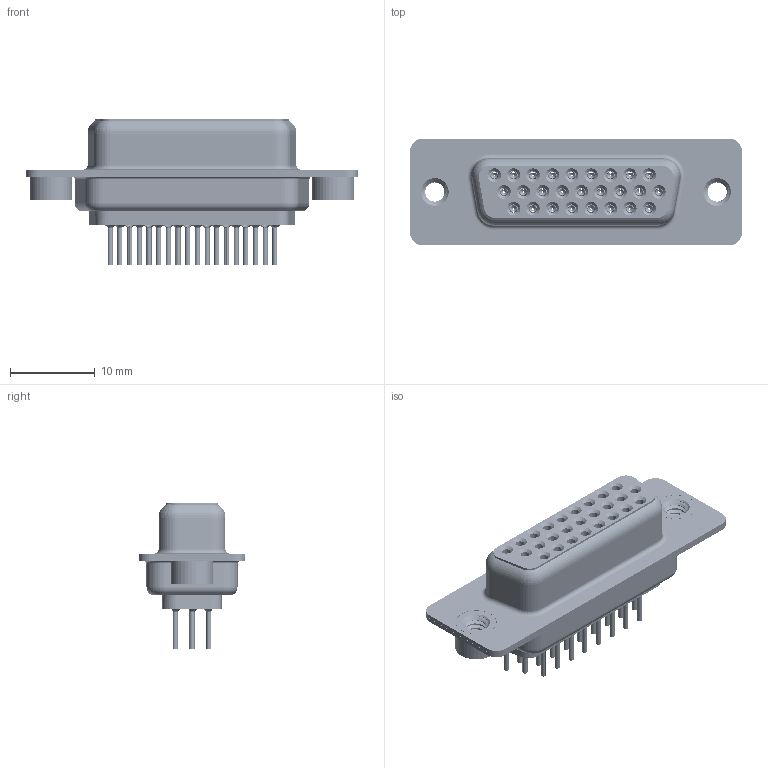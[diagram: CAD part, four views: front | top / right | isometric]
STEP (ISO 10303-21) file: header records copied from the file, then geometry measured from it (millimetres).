
FILE_DESCRIPTION (( 'STEP AP203' ), '1' );
FILE_NAME ('638-026-630-242.STEP', '2020-07-18T21:17:37', ( '' ), ( '' ), 'SwSTEP 2.0', 'SolidWorks 2020', '' );
FILE_SCHEMA (( 'CONFIG_CONTROL_DESIGN' ));
Length unit declared in the file: millimetre
Products named in the file (8): 638 Shell Rear_26 Contacts; 638 Housing_26 Contacts; 638 Contact Row 2_30; 638-026-630-242; 638 4-40 Threaded Rivet; 638 Contact Row 1_30; 638 Contact Row 3_30; 638 Shell Front_26 Contacts
Assembly tree (31 placements, depth 2):
  638-026-630-242
    638 Housing_26 Contacts
    638 Shell Front_26 Contacts
    638 Shell Rear_26 Contacts
    638 Contact Row 1_30  x9
    638 Contact Row 2_30  x9
    638 Contact Row 3_30  x8
    638 4-40 Threaded Rivet  x2
Bounding box: 39.19 x 12.6 x 17.3 mm (x, y, z)
Volume: 2214 mm3; surface area: 8307.2 mm2
Topology: 31 solids, 31 shells, 3581 faces, 9109 edges, 5653 vertices
Faces by surface type: cylinder 995, plane 873, torus 733, bspline 526, cone 454
Entity records: 32767 total; most frequent: CARTESIAN_POINT 9759, DIRECTION 4678, ORIENTED_EDGE 4410, EDGE_CURVE 2205, AXIS2_PLACEMENT_3D 1956, VERTEX_POINT 1386, EDGE_LOOP 1073, CIRCLE 1065
